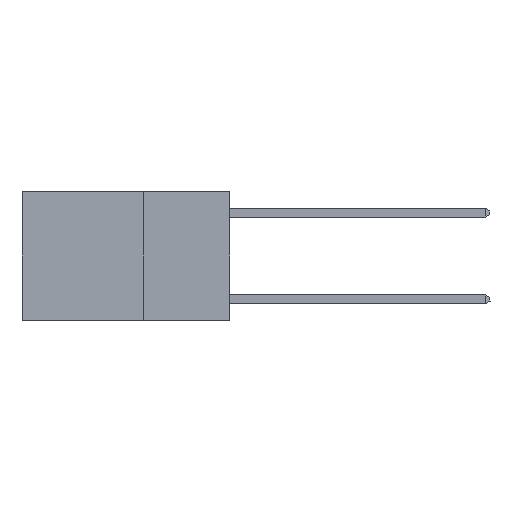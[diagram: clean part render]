
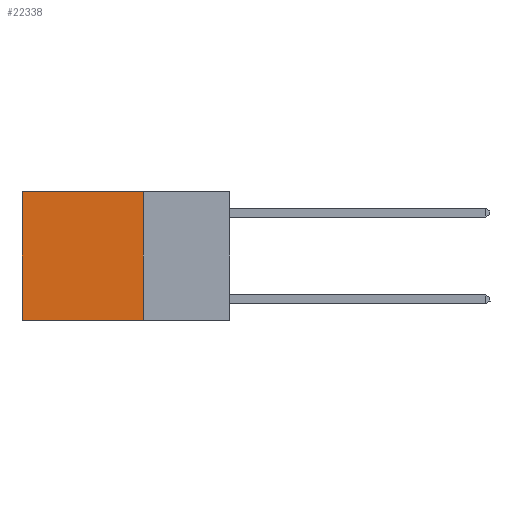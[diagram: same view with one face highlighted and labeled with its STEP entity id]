
A CAD part, left-side view. The second image highlights one B-rep face of the part: STEP entity #22338.
In plain terms, the highlighted planar face has unit normal (-1, 0, 0).
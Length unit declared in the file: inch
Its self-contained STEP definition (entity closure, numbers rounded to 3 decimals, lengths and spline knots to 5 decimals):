
#717 = VERTEX_POINT ( 'NONE', #20495 ) ;
#1367 = PLANE ( 'NONE',  #2727 ) ;
#2727 = AXIS2_PLACEMENT_3D ( 'NONE', #15126, #5519, #5299 ) ;
#5057 = EDGE_LOOP ( 'NONE', ( #21856, #19842, #17854, #26752 ) ) ;
#5144 = FACE_OUTER_BOUND ( 'NONE', #5057, .T. ) ;
#5299 = DIRECTION ( 'NONE',  ( 0., 0., -1. ) ) ;
#5519 = DIRECTION ( 'NONE',  ( 1., 0., 0. ) ) ;
#5636 = DIRECTION ( 'NONE',  ( 0., 1., 0. ) ) ;
#5813 = CARTESIAN_POINT ( 'NONE',  ( 0.2625, 0.6, 0. ) ) ;
#7290 = CARTESIAN_POINT ( 'NONE',  ( 0.2625, 0.6, 0. ) ) ;
#7355 = CARTESIAN_POINT ( 'NONE',  ( 0.2625, 0.25, -0.37 ) ) ;
#8390 = VECTOR ( 'NONE', #26739, 39.37008 ) ;
#9532 = CARTESIAN_POINT ( 'NONE',  ( 0.2625, 0.25, 0. ) ) ;
#9819 = DIRECTION ( 'NONE',  ( 0., 1., 0. ) ) ;
#10019 = VECTOR ( 'NONE', #25791, 39.37008 ) ;
#13434 = EDGE_CURVE ( 'NONE', #19391, #25042, #18372, .T. ) ;
#13713 = LINE ( 'NONE', #7355, #19397 ) ;
#14278 = EDGE_CURVE ( 'NONE', #717, #25042, #13713, .T. ) ;
#14347 = CARTESIAN_POINT ( 'NONE',  ( 0.2625, 0.6, -0.37 ) ) ;
#15126 = CARTESIAN_POINT ( 'NONE',  ( 0.2625, 0.25, 0. ) ) ;
#17751 = CARTESIAN_POINT ( 'NONE',  ( 0.2625, 0.25, 0. ) ) ;
#17854 = ORIENTED_EDGE ( 'NONE', *, *, #18387, .F. ) ;
#18000 = LINE ( 'NONE', #9532, #21782 ) ;
#18372 = LINE ( 'NONE', #7290, #8390 ) ;
#18387 = EDGE_CURVE ( 'NONE', #27249, #717, #19571, .T. ) ;
#19305 = EDGE_CURVE ( 'NONE', #27249, #19391, #18000, .T. ) ;
#19391 = VERTEX_POINT ( 'NONE', #5813 ) ;
#19397 = VECTOR ( 'NONE', #9819, 39.37008 ) ;
#19571 = LINE ( 'NONE', #25564, #10019 ) ;
#19842 = ORIENTED_EDGE ( 'NONE', *, *, #14278, .F. ) ;
#20495 = CARTESIAN_POINT ( 'NONE',  ( 0.2625, 0.25, -0.37 ) ) ;
#21782 = VECTOR ( 'NONE', #5636, 39.37008 ) ;
#21856 = ORIENTED_EDGE ( 'NONE', *, *, #13434, .T. ) ;
#22338 = ADVANCED_FACE ( 'NONE', ( #5144 ), #1367, .F. ) ;
#25042 = VERTEX_POINT ( 'NONE', #14347 ) ;
#25564 = CARTESIAN_POINT ( 'NONE',  ( 0.2625, 0.25, 0. ) ) ;
#25791 = DIRECTION ( 'NONE',  ( 0., 0., -1. ) ) ;
#26739 = DIRECTION ( 'NONE',  ( 0., 0., -1. ) ) ;
#26752 = ORIENTED_EDGE ( 'NONE', *, *, #19305, .T. ) ;
#27249 = VERTEX_POINT ( 'NONE', #17751 ) ;
